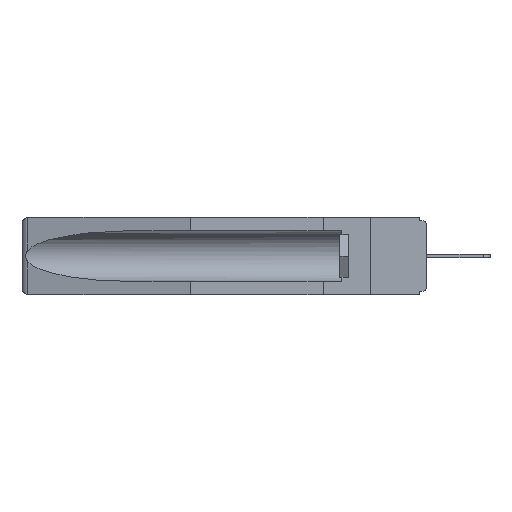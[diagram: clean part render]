
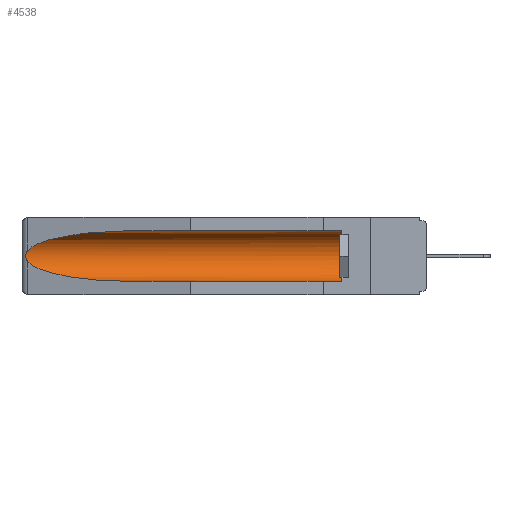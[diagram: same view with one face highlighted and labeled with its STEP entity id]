
A CAD part, left-side view. The second image highlights one B-rep face of the part: STEP entity #4538.
In plain terms, the highlighted cylindrical face has radius 2.857 mm (diameter 5.715 mm), a partial arc.
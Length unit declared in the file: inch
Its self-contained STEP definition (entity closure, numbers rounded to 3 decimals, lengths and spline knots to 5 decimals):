
#201 = CARTESIAN_POINT ( 'NONE',  ( 0.155, 1.07973, -0.284 ) ) ;
#307 = AXIS2_PLACEMENT_3D ( 'NONE', #2328, #21237, #605 ) ;
#605 = DIRECTION ( 'NONE',  ( 0., 0., 1. ) ) ;
#644 = CARTESIAN_POINT ( 'NONE',  ( 0.155, 1.07973, -0.059 ) ) ;
#842 = CARTESIAN_POINT ( 'NONE',  ( 0.26597, 1.52961, -0.15275 ) ) ;
#1300 = ORIENTED_EDGE ( 'NONE', *, *, #18326, .T. ) ;
#1588 = CARTESIAN_POINT ( 'NONE',  ( 0.26537, 1.52718, -0.19328 ) ) ;
#1677 = VERTEX_POINT ( 'NONE', #201 ) ;
#1951 = EDGE_LOOP ( 'NONE', ( #1300, #5701, #7782, #12288, #17771, #15000 ) ) ;
#2328 = CARTESIAN_POINT ( 'NONE',  ( 0.155, 0.126, -0.1715 ) ) ;
#2567 = CARTESIAN_POINT ( 'NONE',  ( 0.2673, 1.5327, -0.16383 ) ) ;
#2866 = CARTESIAN_POINT ( 'NONE',  ( 0.155, 0.126, -0.059 ) ) ;
#2882 = CARTESIAN_POINT ( 'NONE',  ( 0.26537, 1.52718, -0.14972 ) ) ;
#3135 = VECTOR ( 'NONE', #8776, 39.37008 ) ;
#3790 = EDGE_CURVE ( 'NONE', #4447, #4640, #19498, .T. ) ;
#4447 = VERTEX_POINT ( 'NONE', #2866 ) ;
#4538 = ADVANCED_FACE ( 'NONE', ( #12316 ), #6936, .F. ) ;
#4640 = VERTEX_POINT ( 'NONE', #644 ) ;
#4716 = EDGE_CURVE ( 'NONE', #7025, #1677, #16342, .T. ) ;
#5032 = CIRCLE ( 'NONE', #307, 0.1125 ) ;
#5048 = CARTESIAN_POINT ( 'NONE',  ( 0.155, -0.30754, -0.284 ) ) ;
#5238 = DIRECTION ( 'NONE',  ( 0., 1., 0. ) ) ;
#5419 = CARTESIAN_POINT ( 'NONE',  ( 0.21114, 1.30732, -0.284 ) ) ;
#5701 = ORIENTED_EDGE ( 'NONE', *, *, #17968, .T. ) ;
#6831 = CARTESIAN_POINT ( 'NONE',  ( 0.26655, 1.53094, -0.18657 ) ) ;
#6936 = CYLINDRICAL_SURFACE ( 'NONE', #18763, 0.1125 ) ;
#7025 = VERTEX_POINT ( 'NONE', #16477 ) ;
#7782 = ORIENTED_EDGE ( 'NONE', *, *, #4716, .T. ) ;
#8372 = EDGE_CURVE ( 'NONE', #20863, #4447, #5032, .T. ) ;
#8776 = DIRECTION ( 'NONE',  ( 0., 1., 0. ) ) ;
#9928 = CARTESIAN_POINT ( 'NONE',  ( 0.155, 0.126, -0.284 ) ) ;
#10000 = CARTESIAN_POINT ( 'NONE',  ( 0.26537, 1.52718, -0.14972 ) ) ;
#10153 = CARTESIAN_POINT ( 'NONE',  ( 0.26537, 1.52718, -0.14972 ) ) ;
#11171 = CARTESIAN_POINT ( 'NONE',  ( 0.155, 1.07973, -0.059 ) ) ;
#11912 = CARTESIAN_POINT ( 'NONE',  ( 0.155, 1.07973, -0.284 ) ) ;
#12288 = ORIENTED_EDGE ( 'NONE', *, *, #14737, .F. ) ;
#12316 = FACE_OUTER_BOUND ( 'NONE', #1951, .T. ) ;
#13630 = CARTESIAN_POINT ( 'NONE',  ( 0.26537, 1.52718, -0.19328 ) ) ;
#13698 = CARTESIAN_POINT ( 'NONE',  ( 0.26654, 1.53092, -0.15636 ) ) ;
#14186 = LINE ( 'NONE', #5048, #3135 ) ;
#14737 = EDGE_CURVE ( 'NONE', #20863, #1677, #14186, .T. ) ;
#14794 = CARTESIAN_POINT ( 'NONE',  ( 0.155, -0.30754, -0.059 ) ) ;
#15000 = ORIENTED_EDGE ( 'NONE', *, *, #3790, .T. ) ;
#15010 = B_SPLINE_CURVE_WITH_KNOTS ( 'NONE', 3,
 ( #10153, #842, #13698, #2567, #20629, #20016, #15301, #6831, #17224, #1588 ),
 .UNSPECIFIED., .F., .F.,
 ( 4, 2, 2, 2, 4 ),
 ( 0., 0.00029, 0.00058, 0.00087, 0.00117 ),
 .UNSPECIFIED. ) ;
#15271 = CARTESIAN_POINT ( 'NONE',  ( 0.25451, 1.48313, -0.09465 ) ) ;
#15301 = CARTESIAN_POINT ( 'NONE',  ( 0.2673, 1.53269, -0.17917 ) ) ;
#15682 = CARTESIAN_POINT ( 'NONE',  ( 0.25451, 1.48313, -0.24835 ) ) ;
#15966 = DIRECTION ( 'NONE',  ( 0., 0., 1. ) ) ;
#16342 =( BOUNDED_CURVE ( )  B_SPLINE_CURVE ( 3, ( #13630, #15682, #5419, #11912 ),
 .UNSPECIFIED., .F., .F. ) 
 B_SPLINE_CURVE_WITH_KNOTS ( ( 4, 4 ),
 ( 0.1948, 1.5708 ),
 .UNSPECIFIED. ) 
 CURVE ( )  GEOMETRIC_REPRESENTATION_ITEM ( )  RATIONAL_B_SPLINE_CURVE ( ( 1., 0.848, 0.848, 1. ) ) 
 REPRESENTATION_ITEM ( '' )  );
#16439 = CARTESIAN_POINT ( 'NONE',  ( 0.21114, 1.30732, -0.059 ) ) ;
#16477 = CARTESIAN_POINT ( 'NONE',  ( 0.26537, 1.52718, -0.19328 ) ) ;
#17224 = CARTESIAN_POINT ( 'NONE',  ( 0.26597, 1.5296, -0.19026 ) ) ;
#17771 = ORIENTED_EDGE ( 'NONE', *, *, #8372, .T. ) ;
#17968 = EDGE_CURVE ( 'NONE', #19605, #7025, #15010, .T. ) ;
#18326 = EDGE_CURVE ( 'NONE', #4640, #19605, #20823, .T. ) ;
#18763 = AXIS2_PLACEMENT_3D ( 'NONE', #19279, #5238, #15966 ) ;
#19279 = CARTESIAN_POINT ( 'NONE',  ( 0.155, -0.30754, -0.1715 ) ) ;
#19498 = LINE ( 'NONE', #14794, #20855 ) ;
#19605 = VERTEX_POINT ( 'NONE', #2882 ) ;
#20016 = CARTESIAN_POINT ( 'NONE',  ( 0.2675, 1.53308, -0.17534 ) ) ;
#20629 = CARTESIAN_POINT ( 'NONE',  ( 0.2675, 1.53308, -0.16763 ) ) ;
#20823 =( BOUNDED_CURVE ( )  B_SPLINE_CURVE ( 3, ( #11171, #16439, #15271, #10000 ),
 .UNSPECIFIED., .F., .F. ) 
 B_SPLINE_CURVE_WITH_KNOTS ( ( 4, 4 ),
 ( 4.71239, 6.08839 ),
 .UNSPECIFIED. ) 
 CURVE ( )  GEOMETRIC_REPRESENTATION_ITEM ( )  RATIONAL_B_SPLINE_CURVE ( ( 1., 0.848, 0.848, 1. ) ) 
 REPRESENTATION_ITEM ( '' )  );
#20855 = VECTOR ( 'NONE', #21525, 39.37008 ) ;
#20863 = VERTEX_POINT ( 'NONE', #9928 ) ;
#21237 = DIRECTION ( 'NONE',  ( 0., -1., 0. ) ) ;
#21525 = DIRECTION ( 'NONE',  ( 0., 1., 0. ) ) ;
